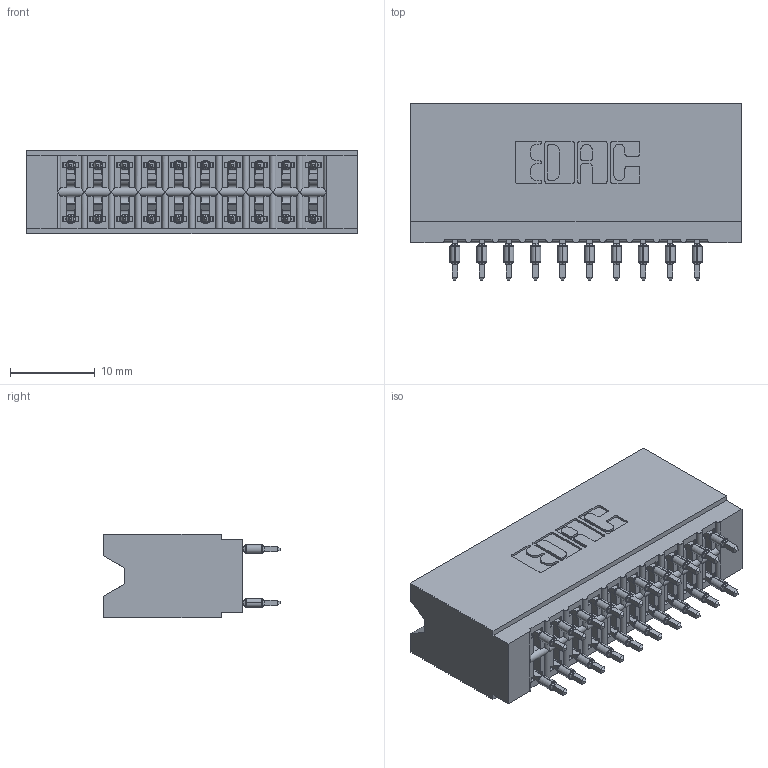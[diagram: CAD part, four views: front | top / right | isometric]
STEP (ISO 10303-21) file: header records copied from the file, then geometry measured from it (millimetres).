
FILE_DESCRIPTION (( 'STEP AP203' ), '1' );
FILE_NAME ('746-020-560-206.STEP', '2026-02-26T22:28:15', ( '' ), ( '' ), 'SwSTEP 2.0', 'SolidWorks 2023', '' );
FILE_SCHEMA (( 'CONFIG_CONTROL_DESIGN' ));
Length unit declared in the file: millimetre
Products named in the file (3): 746-292-001_560; 746 Part_.515 Slot Depth - 06; 746-020-560-206
Assembly tree (21 placements, depth 2):
  746-020-560-206
    746 Part_.515 Slot Depth - 06
    746-292-001_560  x20
Bounding box: 38.99 x 20.82 x 9.91 mm (x, y, z)
Volume: 4431.5 mm3; surface area: 6818.4 mm2
Topology: 21 solids, 21 shells, 1988 faces, 5525 edges, 3545 vertices
Faces by surface type: plane 996, cylinder 472, bspline 400, torus 120
Entity records: 20156 total; most frequent: CARTESIAN_POINT 4282, ORIENTED_EDGE 3374, DIRECTION 2879, EDGE_CURVE 1687, VECTOR 1395, LINE 1395, VERTEX_POINT 1113, AXIS2_PLACEMENT_3D 742
